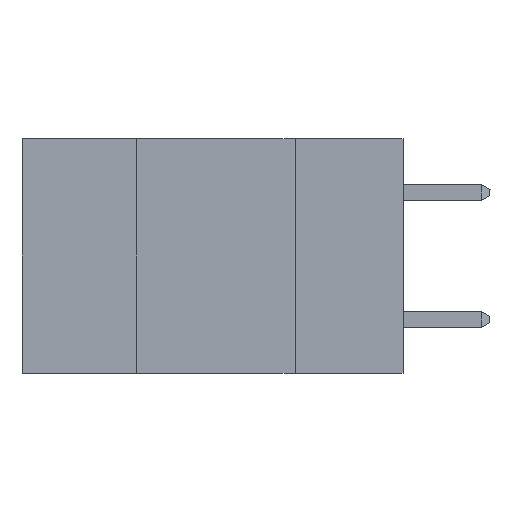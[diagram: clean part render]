
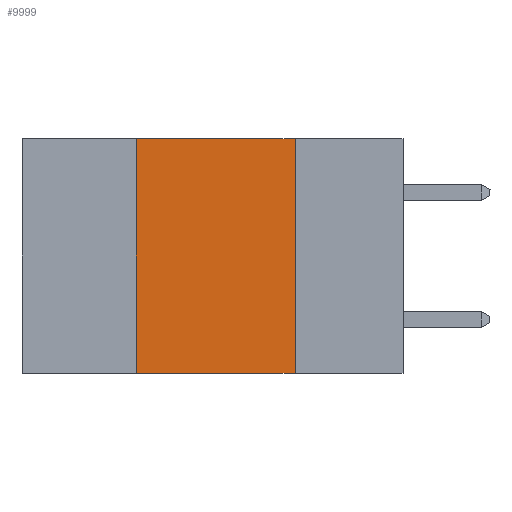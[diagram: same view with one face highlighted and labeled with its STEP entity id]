
A CAD part, left-side view. The second image highlights one B-rep face of the part: STEP entity #9999.
In plain terms, the highlighted planar face has unit normal (-1, 0, 0).
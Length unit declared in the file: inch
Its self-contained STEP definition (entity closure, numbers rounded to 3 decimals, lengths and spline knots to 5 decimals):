
#984 = EDGE_CURVE ( 'NONE', #7263, #5546, #1217, .T. ) ;
#1007 = CARTESIAN_POINT ( 'NONE',  ( 0., 0.17, 0. ) ) ;
#1217 = LINE ( 'NONE', #1232, #11442 ) ;
#1232 = CARTESIAN_POINT ( 'NONE',  ( 0., 0.6, 0. ) ) ;
#1450 = DIRECTION ( 'NONE',  ( 1., 0., 0. ) ) ;
#1774 = VECTOR ( 'NONE', #12141, 39.37008 ) ;
#2015 = ORIENTED_EDGE ( 'NONE', *, *, #5535, .F. ) ;
#2039 = CARTESIAN_POINT ( 'NONE',  ( 0., 0.17, 0. ) ) ;
#2581 = LINE ( 'NONE', #5423, #7169 ) ;
#3261 = PLANE ( 'NONE',  #6911 ) ;
#4031 = VERTEX_POINT ( 'NONE', #6633 ) ;
#4585 = FACE_OUTER_BOUND ( 'NONE', #9025, .T. ) ;
#4699 = VECTOR ( 'NONE', #9919, 39.37008 ) ;
#5293 = EDGE_CURVE ( 'NONE', #4031, #7263, #2581, .T. ) ;
#5303 = LINE ( 'NONE', #1007, #4699 ) ;
#5423 = CARTESIAN_POINT ( 'NONE',  ( 0., 0.42, 0. ) ) ;
#5535 = EDGE_CURVE ( 'NONE', #5546, #6324, #5303, .T. ) ;
#5546 = VERTEX_POINT ( 'NONE', #2039 ) ;
#6324 = VERTEX_POINT ( 'NONE', #12727 ) ;
#6633 = CARTESIAN_POINT ( 'NONE',  ( 0., 0.42, -0.37 ) ) ;
#6911 = AXIS2_PLACEMENT_3D ( 'NONE', #9235, #1450, #8365 ) ;
#7169 = VECTOR ( 'NONE', #12408, 39.37008 ) ;
#7246 = ORIENTED_EDGE ( 'NONE', *, *, #984, .F. ) ;
#7263 = VERTEX_POINT ( 'NONE', #11033 ) ;
#8365 = DIRECTION ( 'NONE',  ( 0., 0., -1. ) ) ;
#8398 = LINE ( 'NONE', #9225, #1774 ) ;
#8572 = ORIENTED_EDGE ( 'NONE', *, *, #5293, .F. ) ;
#9025 = EDGE_LOOP ( 'NONE', ( #2015, #7246, #8572, #11269 ) ) ;
#9099 = DIRECTION ( 'NONE',  ( 0., -1., 0. ) ) ;
#9225 = CARTESIAN_POINT ( 'NONE',  ( 0., 0.6, -0.37 ) ) ;
#9235 = CARTESIAN_POINT ( 'NONE',  ( 0., 0.6, 0. ) ) ;
#9919 = DIRECTION ( 'NONE',  ( 0., 0., -1. ) ) ;
#9999 = ADVANCED_FACE ( 'NONE', ( #4585 ), #3261, .F. ) ;
#11033 = CARTESIAN_POINT ( 'NONE',  ( 0., 0.42, 0. ) ) ;
#11269 = ORIENTED_EDGE ( 'NONE', *, *, #12467, .T. ) ;
#11442 = VECTOR ( 'NONE', #9099, 39.37008 ) ;
#12141 = DIRECTION ( 'NONE',  ( 0., -1., 0. ) ) ;
#12408 = DIRECTION ( 'NONE',  ( 0., 0., 1. ) ) ;
#12467 = EDGE_CURVE ( 'NONE', #4031, #6324, #8398, .T. ) ;
#12727 = CARTESIAN_POINT ( 'NONE',  ( 0., 0.17, -0.37 ) ) ;
